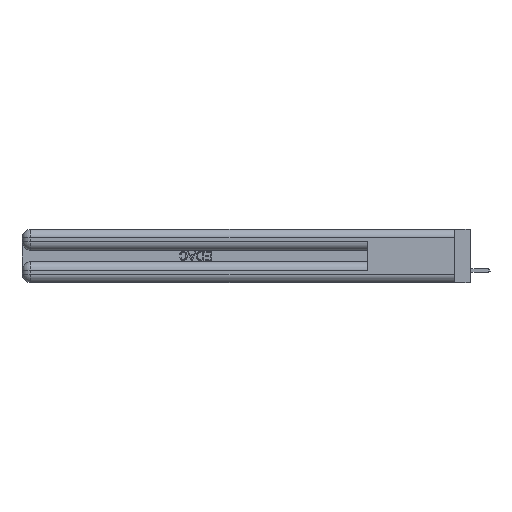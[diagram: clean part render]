
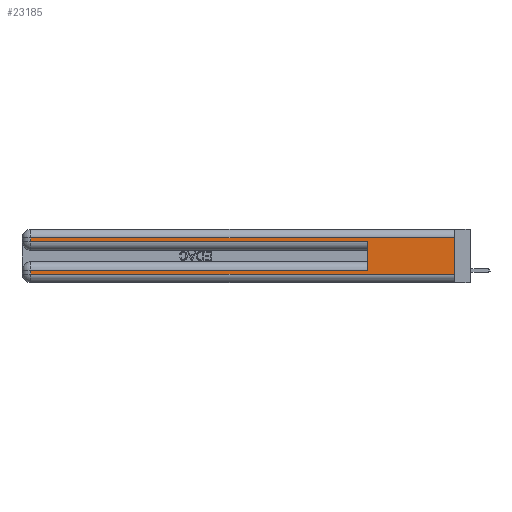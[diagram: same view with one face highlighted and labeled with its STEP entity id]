
A CAD part, left-side view. The second image highlights one B-rep face of the part: STEP entity #23185.
In plain terms, the highlighted planar face has unit normal (-1, 0, 0).
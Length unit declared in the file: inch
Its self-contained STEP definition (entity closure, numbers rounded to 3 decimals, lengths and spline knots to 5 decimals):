
#421 = DIRECTION ( 'NONE',  ( 0., 0., -1. ) ) ;
#1096 = EDGE_LOOP ( 'NONE', ( #28972, #38155, #19189, #27627, #17658, #26348, #38306, #12777 ) ) ;
#1235 = EDGE_CURVE ( 'NONE', #10244, #30665, #27629, .T. ) ;
#1647 = VECTOR ( 'NONE', #19009, 39.37008 ) ;
#1753 = EDGE_CURVE ( 'NONE', #38484, #8541, #10568, .T. ) ;
#3886 = CARTESIAN_POINT ( 'NONE',  ( 0., 2.94, 0.37 ) ) ;
#4443 = CARTESIAN_POINT ( 'NONE',  ( 0., 0.6, 0.145 ) ) ;
#4596 = VECTOR ( 'NONE', #7104, 39.37008 ) ;
#6297 = VECTOR ( 'NONE', #18047, 39.37008 ) ;
#7104 = DIRECTION ( 'NONE',  ( 0., 0., -1. ) ) ;
#8071 = DIRECTION ( 'NONE',  ( 0., -1., 0. ) ) ;
#8184 = PLANE ( 'NONE',  #15294 ) ;
#8242 = DIRECTION ( 'NONE',  ( 0., 1., 0. ) ) ;
#8409 = CARTESIAN_POINT ( 'NONE',  ( 0., 2.94, 0.285 ) ) ;
#8516 = CARTESIAN_POINT ( 'NONE',  ( 0., 0.6, 0.085 ) ) ;
#8541 = VERTEX_POINT ( 'NONE', #17830 ) ;
#8638 = VERTEX_POINT ( 'NONE', #8516 ) ;
#10244 = VERTEX_POINT ( 'NONE', #35518 ) ;
#10568 = LINE ( 'NONE', #3886, #4596 ) ;
#11609 = CARTESIAN_POINT ( 'NONE',  ( 0., 2.94, 0.31 ) ) ;
#12777 = ORIENTED_EDGE ( 'NONE', *, *, #17393, .T. ) ;
#14103 = CARTESIAN_POINT ( 'NONE',  ( 0., 0., 0.37 ) ) ;
#14242 = CARTESIAN_POINT ( 'NONE',  ( 0., 0., 0.06 ) ) ;
#15294 = AXIS2_PLACEMENT_3D ( 'NONE', #22844, #35463, #421 ) ;
#15670 = LINE ( 'NONE', #23824, #18666 ) ;
#15689 = CARTESIAN_POINT ( 'NONE',  ( 0., 2.94, 0.085 ) ) ;
#16116 = VECTOR ( 'NONE', #26440, 39.37008 ) ;
#17283 = VERTEX_POINT ( 'NONE', #8409 ) ;
#17306 = VERTEX_POINT ( 'NONE', #11609 ) ;
#17393 = EDGE_CURVE ( 'NONE', #8541, #30665, #15670, .T. ) ;
#17658 = ORIENTED_EDGE ( 'NONE', *, *, #23550, .F. ) ;
#17830 = CARTESIAN_POINT ( 'NONE',  ( 0., 2.94, 0.06 ) ) ;
#18047 = DIRECTION ( 'NONE',  ( 0., -1., 0. ) ) ;
#18666 = VECTOR ( 'NONE', #8071, 39.37008 ) ;
#19009 = DIRECTION ( 'NONE',  ( 0., 1., 0. ) ) ;
#19189 = ORIENTED_EDGE ( 'NONE', *, *, #23020, .T. ) ;
#21470 = CARTESIAN_POINT ( 'NONE',  ( 0., 0., 0.31 ) ) ;
#21639 = LINE ( 'NONE', #4443, #16116 ) ;
#22240 = CARTESIAN_POINT ( 'NONE',  ( 0., 0.6, 0.285 ) ) ;
#22364 = EDGE_CURVE ( 'NONE', #10244, #17306, #27806, .T. ) ;
#22666 = LINE ( 'NONE', #33841, #6297 ) ;
#22844 = CARTESIAN_POINT ( 'NONE',  ( 0., 0., 0.37 ) ) ;
#23020 = EDGE_CURVE ( 'NONE', #17306, #17283, #36721, .T. ) ;
#23185 = ADVANCED_FACE ( 'NONE', ( #35660 ), #8184, .F. ) ;
#23550 = EDGE_CURVE ( 'NONE', #8638, #28750, #21639, .T. ) ;
#23760 = VECTOR ( 'NONE', #8242, 39.37008 ) ;
#23824 = CARTESIAN_POINT ( 'NONE',  ( 0., 0., 0.06 ) ) ;
#24116 = VECTOR ( 'NONE', #39910, 39.37008 ) ;
#26348 = ORIENTED_EDGE ( 'NONE', *, *, #33449, .T. ) ;
#26440 = DIRECTION ( 'NONE',  ( 0., 0., 1. ) ) ;
#27627 = ORIENTED_EDGE ( 'NONE', *, *, #38341, .T. ) ;
#27629 = LINE ( 'NONE', #14103, #24116 ) ;
#27806 = LINE ( 'NONE', #21470, #23760 ) ;
#28023 = CARTESIAN_POINT ( 'NONE',  ( 0., 2.94, 0.37 ) ) ;
#28146 = LINE ( 'NONE', #34820, #1647 ) ;
#28264 = VECTOR ( 'NONE', #40940, 39.37008 ) ;
#28750 = VERTEX_POINT ( 'NONE', #22240 ) ;
#28972 = ORIENTED_EDGE ( 'NONE', *, *, #1235, .F. ) ;
#30665 = VERTEX_POINT ( 'NONE', #14242 ) ;
#33449 = EDGE_CURVE ( 'NONE', #8638, #38484, #28146, .T. ) ;
#33841 = CARTESIAN_POINT ( 'NONE',  ( 0., 0., 0.285 ) ) ;
#34820 = CARTESIAN_POINT ( 'NONE',  ( 0., 0., 0.085 ) ) ;
#35463 = DIRECTION ( 'NONE',  ( 1., 0., 0. ) ) ;
#35518 = CARTESIAN_POINT ( 'NONE',  ( 0., 0., 0.31 ) ) ;
#35660 = FACE_OUTER_BOUND ( 'NONE', #1096, .T. ) ;
#36721 = LINE ( 'NONE', #28023, #28264 ) ;
#38155 = ORIENTED_EDGE ( 'NONE', *, *, #22364, .T. ) ;
#38306 = ORIENTED_EDGE ( 'NONE', *, *, #1753, .T. ) ;
#38341 = EDGE_CURVE ( 'NONE', #17283, #28750, #22666, .T. ) ;
#38484 = VERTEX_POINT ( 'NONE', #15689 ) ;
#39910 = DIRECTION ( 'NONE',  ( 0., 0., -1. ) ) ;
#40940 = DIRECTION ( 'NONE',  ( 0., 0., -1. ) ) ;
